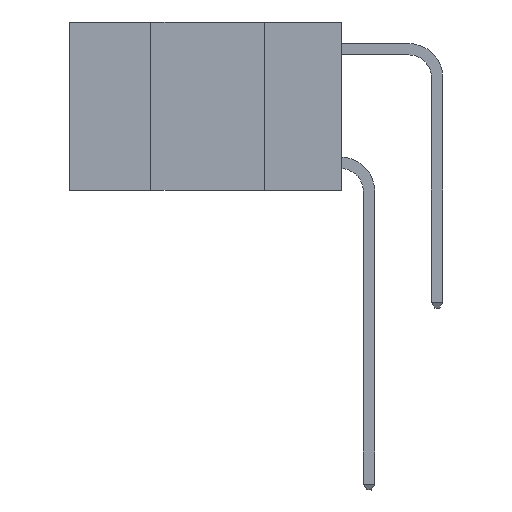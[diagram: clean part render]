
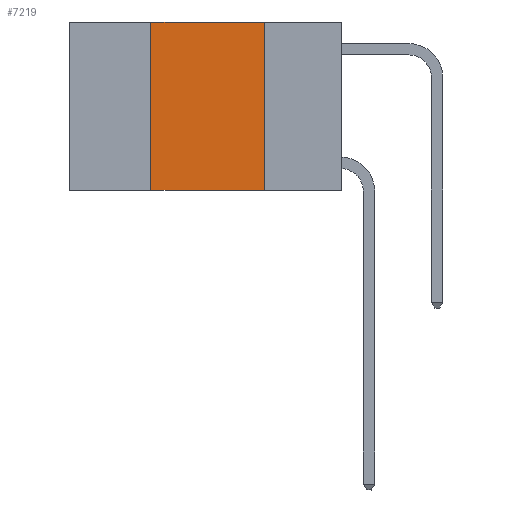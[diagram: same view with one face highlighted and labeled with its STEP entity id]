
A CAD part, left-side view. The second image highlights one B-rep face of the part: STEP entity #7219.
In plain terms, the highlighted planar face has unit normal (-1, 0, 0).
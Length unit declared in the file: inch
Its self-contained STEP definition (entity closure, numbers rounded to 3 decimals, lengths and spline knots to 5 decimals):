
#101 = LINE ( 'NONE', #16593, #1606 ) ;
#1003 = DIRECTION ( 'NONE',  ( 0., 0., -1. ) ) ;
#1407 = PLANE ( 'NONE',  #5750 ) ;
#1606 = VECTOR ( 'NONE', #3022, 39.37008 ) ;
#1805 = DIRECTION ( 'NONE',  ( 0., -1., 0. ) ) ;
#2376 = VERTEX_POINT ( 'NONE', #18471 ) ;
#2975 = EDGE_LOOP ( 'NONE', ( #14367, #9174, #9142, #14877 ) ) ;
#3022 = DIRECTION ( 'NONE',  ( 0., 0., 1. ) ) ;
#3439 = EDGE_CURVE ( 'NONE', #8249, #24430, #22369, .T. ) ;
#5750 = AXIS2_PLACEMENT_3D ( 'NONE', #24000, #12554, #15230 ) ;
#5940 = VECTOR ( 'NONE', #1003, 39.37008 ) ;
#5973 = VECTOR ( 'NONE', #1805, 39.37008 ) ;
#6788 = EDGE_CURVE ( 'NONE', #15560, #2376, #101, .T. ) ;
#7219 = ADVANCED_FACE ( 'NONE', ( #22731 ), #1407, .F. ) ;
#7772 = DIRECTION ( 'NONE',  ( 0., -1., 0. ) ) ;
#8249 = VERTEX_POINT ( 'NONE', #16186 ) ;
#9142 = ORIENTED_EDGE ( 'NONE', *, *, #6788, .F. ) ;
#9174 = ORIENTED_EDGE ( 'NONE', *, *, #22588, .F. ) ;
#11531 = CARTESIAN_POINT ( 'NONE',  ( 0., 0.6, -0.37 ) ) ;
#11836 = CARTESIAN_POINT ( 'NONE',  ( 0., 0.17, -0.37 ) ) ;
#12554 = DIRECTION ( 'NONE',  ( 1., 0., 0. ) ) ;
#12782 = CARTESIAN_POINT ( 'NONE',  ( 0., 0.42, -0.37 ) ) ;
#13937 = VECTOR ( 'NONE', #7772, 39.37008 ) ;
#14367 = ORIENTED_EDGE ( 'NONE', *, *, #3439, .F. ) ;
#14877 = ORIENTED_EDGE ( 'NONE', *, *, #18953, .T. ) ;
#15230 = DIRECTION ( 'NONE',  ( 0., 0., -1. ) ) ;
#15560 = VERTEX_POINT ( 'NONE', #12782 ) ;
#16186 = CARTESIAN_POINT ( 'NONE',  ( 0., 0.17, 0. ) ) ;
#16320 = LINE ( 'NONE', #11531, #13937 ) ;
#16593 = CARTESIAN_POINT ( 'NONE',  ( 0., 0.42, 0. ) ) ;
#17594 = LINE ( 'NONE', #22792, #5973 ) ;
#18471 = CARTESIAN_POINT ( 'NONE',  ( 0., 0.42, 0. ) ) ;
#18953 = EDGE_CURVE ( 'NONE', #15560, #24430, #16320, .T. ) ;
#20087 = CARTESIAN_POINT ( 'NONE',  ( 0., 0.17, 0. ) ) ;
#22369 = LINE ( 'NONE', #20087, #5940 ) ;
#22588 = EDGE_CURVE ( 'NONE', #2376, #8249, #17594, .T. ) ;
#22731 = FACE_OUTER_BOUND ( 'NONE', #2975, .T. ) ;
#22792 = CARTESIAN_POINT ( 'NONE',  ( 0., 0.6, 0. ) ) ;
#24000 = CARTESIAN_POINT ( 'NONE',  ( 0., 0.6, 0. ) ) ;
#24430 = VERTEX_POINT ( 'NONE', #11836 ) ;
